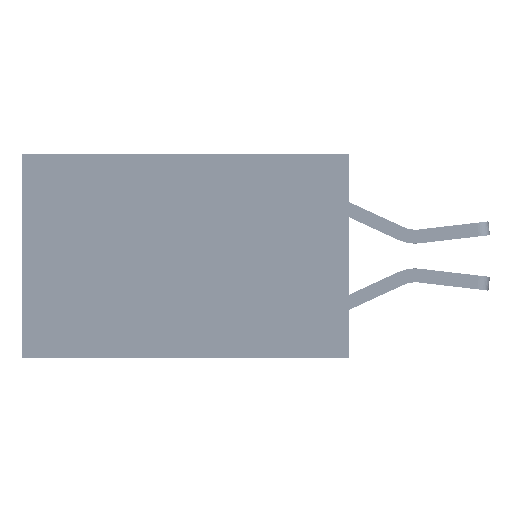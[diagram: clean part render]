
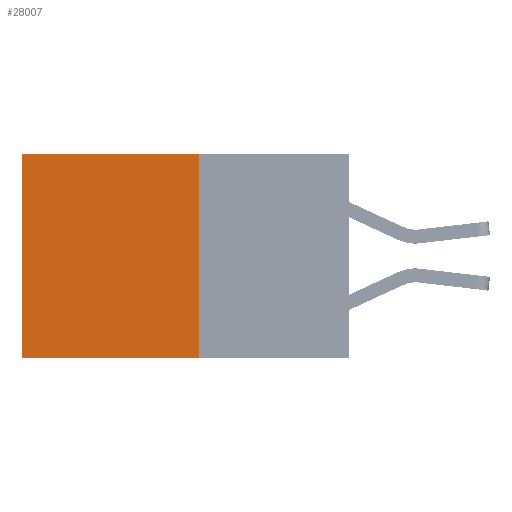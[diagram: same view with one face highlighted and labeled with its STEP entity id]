
A CAD part, left-side view. The second image highlights one B-rep face of the part: STEP entity #28007.
In plain terms, the highlighted planar face has unit normal (-1, 0, 0).
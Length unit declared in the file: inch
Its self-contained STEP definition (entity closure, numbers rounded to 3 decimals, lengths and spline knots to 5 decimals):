
#8 = CARTESIAN_POINT ( 'NONE',  ( 0.277, 0.59, -0.37 ) ) ;
#172 = CARTESIAN_POINT ( 'NONE',  ( 0.277, 0.27, -0.37 ) ) ;
#240 = DIRECTION ( 'NONE',  ( 0., 0., -1. ) ) ;
#543 = VECTOR ( 'NONE', #18762, 39.37008 ) ;
#1853 = EDGE_CURVE ( 'NONE', #9307, #16784, #21110, .T. ) ;
#3748 = AXIS2_PLACEMENT_3D ( 'NONE', #172, #20797, #5322 ) ;
#4049 = ORIENTED_EDGE ( 'NONE', *, *, #5666, .T. ) ;
#4700 = ORIENTED_EDGE ( 'NONE', *, *, #1853, .F. ) ;
#5125 = LINE ( 'NONE', #6954, #12788 ) ;
#5209 = FACE_OUTER_BOUND ( 'NONE', #14131, .T. ) ;
#5322 = DIRECTION ( 'NONE',  ( 0., 0., -1. ) ) ;
#5666 = EDGE_CURVE ( 'NONE', #30799, #17933, #31454, .T. ) ;
#6535 = ORIENTED_EDGE ( 'NONE', *, *, #29270, .T. ) ;
#6954 = CARTESIAN_POINT ( 'NONE',  ( 0.277, 0.27, 0. ) ) ;
#7845 = VECTOR ( 'NONE', #19809, 39.37008 ) ;
#9307 = VERTEX_POINT ( 'NONE', #19755 ) ;
#10282 = LINE ( 'NONE', #17198, #7845 ) ;
#12125 = DIRECTION ( 'NONE',  ( 0., 1., 0. ) ) ;
#12788 = VECTOR ( 'NONE', #12125, 39.37008 ) ;
#12985 = PLANE ( 'NONE',  #3748 ) ;
#13054 = CARTESIAN_POINT ( 'NONE',  ( 0.277, 0.59, 0. ) ) ;
#14131 = EDGE_LOOP ( 'NONE', ( #4049, #25773, #4700, #6535 ) ) ;
#16784 = VERTEX_POINT ( 'NONE', #32536 ) ;
#17198 = CARTESIAN_POINT ( 'NONE',  ( 0.277, 0.27, -0.37 ) ) ;
#17933 = VERTEX_POINT ( 'NONE', #29133 ) ;
#18606 = CARTESIAN_POINT ( 'NONE',  ( 0.277, 0.27, -0.37 ) ) ;
#18762 = DIRECTION ( 'NONE',  ( 0., 0., -1. ) ) ;
#19755 = CARTESIAN_POINT ( 'NONE',  ( 0.277, 0.27, 0. ) ) ;
#19809 = DIRECTION ( 'NONE',  ( 0., 1., 0. ) ) ;
#20797 = DIRECTION ( 'NONE',  ( 1., 0., 0. ) ) ;
#21110 = LINE ( 'NONE', #18606, #543 ) ;
#24931 = VECTOR ( 'NONE', #240, 39.37008 ) ;
#25272 = EDGE_CURVE ( 'NONE', #16784, #17933, #10282, .T. ) ;
#25773 = ORIENTED_EDGE ( 'NONE', *, *, #25272, .F. ) ;
#28007 = ADVANCED_FACE ( 'NONE', ( #5209 ), #12985, .F. ) ;
#29133 = CARTESIAN_POINT ( 'NONE',  ( 0.277, 0.59, -0.37 ) ) ;
#29270 = EDGE_CURVE ( 'NONE', #9307, #30799, #5125, .T. ) ;
#30799 = VERTEX_POINT ( 'NONE', #13054 ) ;
#31454 = LINE ( 'NONE', #8, #24931 ) ;
#32536 = CARTESIAN_POINT ( 'NONE',  ( 0.277, 0.27, -0.37 ) ) ;
